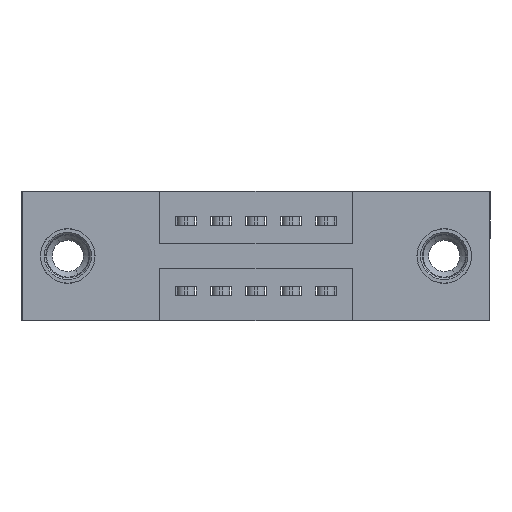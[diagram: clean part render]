
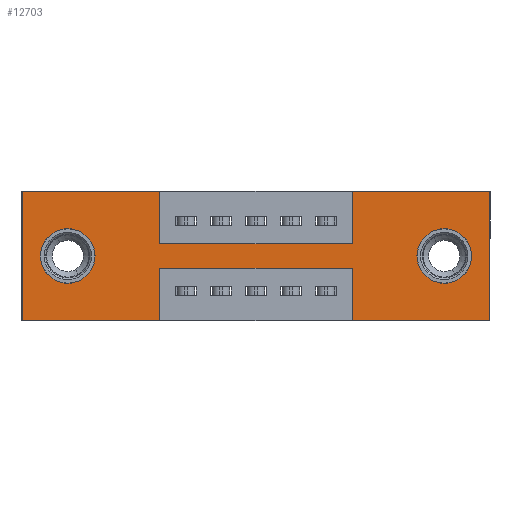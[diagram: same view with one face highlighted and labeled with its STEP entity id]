
A CAD part, front view. The second image highlights one B-rep face of the part: STEP entity #12703.
In plain terms, the highlighted planar face has unit normal (0, -1, 0).
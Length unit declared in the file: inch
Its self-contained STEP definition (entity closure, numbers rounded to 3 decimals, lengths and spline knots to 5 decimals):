
#66 = ORIENTED_EDGE ( 'NONE', *, *, #3494, .F. ) ;
#139 = LINE ( 'NONE', #12505, #10980 ) ;
#207 = DIRECTION ( 'NONE',  ( 0., 1., 0. ) ) ;
#402 = CARTESIAN_POINT ( 'NONE',  ( 0.3925, 0., -0.15 ) ) ;
#464 = ORIENTED_EDGE ( 'NONE', *, *, #2959, .T. ) ;
#584 = CARTESIAN_POINT ( 'NONE',  ( 0., 0., 0. ) ) ;
#816 = CARTESIAN_POINT ( 'NONE',  ( 1.335, 0., -0.37 ) ) ;
#910 = VECTOR ( 'NONE', #1062, 39.37008 ) ;
#927 = LINE ( 'NONE', #5054, #3388 ) ;
#940 = VERTEX_POINT ( 'NONE', #6028 ) ;
#985 = DIRECTION ( 'NONE',  ( 0., 0., -1. ) ) ;
#1062 = DIRECTION ( 'NONE',  ( -1., 0., 0. ) ) ;
#1166 = DIRECTION ( 'NONE',  ( 1., 0., 0. ) ) ;
#1214 = CIRCLE ( 'NONE', #7462, 0.078 ) ;
#1317 = EDGE_CURVE ( 'NONE', #9127, #8757, #927, .T. ) ;
#1395 = VECTOR ( 'NONE', #6409, 39.37008 ) ;
#1417 = VERTEX_POINT ( 'NONE', #12292 ) ;
#1451 = EDGE_CURVE ( 'NONE', #7042, #5371, #3368, .T. ) ;
#1458 = FACE_BOUND ( 'NONE', #3312, .T. ) ;
#1490 = CARTESIAN_POINT ( 'NONE',  ( 1.335, 0., 0. ) ) ;
#1551 = AXIS2_PLACEMENT_3D ( 'NONE', #11576, #4367, #9561 ) ;
#1756 = DIRECTION ( 'NONE',  ( 0., 0., -1. ) ) ;
#1987 = VERTEX_POINT ( 'NONE', #10282 ) ;
#2015 = ORIENTED_EDGE ( 'NONE', *, *, #8600, .F. ) ;
#2095 = VERTEX_POINT ( 'NONE', #2300 ) ;
#2158 = EDGE_CURVE ( 'NONE', #5371, #1417, #6440, .T. ) ;
#2300 = CARTESIAN_POINT ( 'NONE',  ( 0., 0., -0.37 ) ) ;
#2510 = VECTOR ( 'NONE', #7547, 39.37008 ) ;
#2517 = ORIENTED_EDGE ( 'NONE', *, *, #7782, .F. ) ;
#2550 = ORIENTED_EDGE ( 'NONE', *, *, #2588, .F. ) ;
#2588 = EDGE_CURVE ( 'NONE', #3691, #11676, #3673, .T. ) ;
#2832 = CARTESIAN_POINT ( 'NONE',  ( 1.205, 0., -0.107 ) ) ;
#2907 = CARTESIAN_POINT ( 'NONE',  ( 1.205, 0., -0.185 ) ) ;
#2959 = EDGE_CURVE ( 'NONE', #940, #1987, #1214, .T. ) ;
#3046 = VECTOR ( 'NONE', #7233, 39.37008 ) ;
#3155 = VECTOR ( 'NONE', #13037, 39.37008 ) ;
#3312 = EDGE_LOOP ( 'NONE', ( #464, #8197 ) ) ;
#3368 = LINE ( 'NONE', #5937, #8579 ) ;
#3388 = VECTOR ( 'NONE', #12450, 39.37008 ) ;
#3494 = EDGE_CURVE ( 'NONE', #8757, #12376, #10545, .T. ) ;
#3605 = LINE ( 'NONE', #10499, #11149 ) ;
#3608 = EDGE_CURVE ( 'NONE', #6012, #10564, #13182, .T. ) ;
#3673 = LINE ( 'NONE', #12745, #1395 ) ;
#3691 = VERTEX_POINT ( 'NONE', #12827 ) ;
#3743 = PLANE ( 'NONE',  #10872 ) ;
#3776 = VERTEX_POINT ( 'NONE', #2832 ) ;
#3881 = EDGE_CURVE ( 'NONE', #11676, #6012, #12676, .T. ) ;
#4076 = CARTESIAN_POINT ( 'NONE',  ( 1.205, 0., -0.185 ) ) ;
#4189 = DIRECTION ( 'NONE',  ( -1., 0., 0. ) ) ;
#4218 = FACE_BOUND ( 'NONE', #6332, .T. ) ;
#4247 = AXIS2_PLACEMENT_3D ( 'NONE', #4076, #12388, #6031 ) ;
#4367 = DIRECTION ( 'NONE',  ( 0., 1., 0. ) ) ;
#4570 = ORIENTED_EDGE ( 'NONE', *, *, #5522, .F. ) ;
#4667 = EDGE_CURVE ( 'NONE', #5597, #3776, #7029, .T. ) ;
#4749 = DIRECTION ( 'NONE',  ( 0., 0., 1. ) ) ;
#4800 = ORIENTED_EDGE ( 'NONE', *, *, #10953, .T. ) ;
#5054 = CARTESIAN_POINT ( 'NONE',  ( 0.3925, 0., -0.22 ) ) ;
#5285 = CARTESIAN_POINT ( 'NONE',  ( 0.9425, 0., -0.15 ) ) ;
#5371 = VERTEX_POINT ( 'NONE', #816 ) ;
#5380 = CIRCLE ( 'NONE', #1551, 0.078 ) ;
#5448 = VECTOR ( 'NONE', #12685, 39.37008 ) ;
#5522 = EDGE_CURVE ( 'NONE', #12376, #2095, #3605, .T. ) ;
#5597 = VERTEX_POINT ( 'NONE', #5652 ) ;
#5652 = CARTESIAN_POINT ( 'NONE',  ( 1.205, 0., -0.263 ) ) ;
#5726 = LINE ( 'NONE', #7414, #12493 ) ;
#5830 = DIRECTION ( 'NONE',  ( 0., -1., 0. ) ) ;
#5933 = EDGE_CURVE ( 'NONE', #1417, #9127, #139, .T. ) ;
#5937 = CARTESIAN_POINT ( 'NONE',  ( 1.335, 0., 0. ) ) ;
#5967 = EDGE_CURVE ( 'NONE', #1987, #940, #5380, .T. ) ;
#6012 = VERTEX_POINT ( 'NONE', #5285 ) ;
#6028 = CARTESIAN_POINT ( 'NONE',  ( 0.13, 0., -0.107 ) ) ;
#6031 = DIRECTION ( 'NONE',  ( 0., 0., -1. ) ) ;
#6054 = ORIENTED_EDGE ( 'NONE', *, *, #1451, .F. ) ;
#6133 = LINE ( 'NONE', #584, #11917 ) ;
#6138 = DIRECTION ( 'NONE',  ( 0., 0., 1. ) ) ;
#6332 = EDGE_LOOP ( 'NONE', ( #4800, #13461 ) ) ;
#6362 = CARTESIAN_POINT ( 'NONE',  ( 0.9425, 0., 0. ) ) ;
#6409 = DIRECTION ( 'NONE',  ( 0., 0., -1. ) ) ;
#6440 = LINE ( 'NONE', #10510, #910 ) ;
#7029 = CIRCLE ( 'NONE', #4247, 0.078 ) ;
#7042 = VERTEX_POINT ( 'NONE', #1490 ) ;
#7233 = DIRECTION ( 'NONE',  ( 1., 0., 0. ) ) ;
#7251 = ORIENTED_EDGE ( 'NONE', *, *, #2158, .F. ) ;
#7397 = CARTESIAN_POINT ( 'NONE',  ( 0.3925, 0., -0.15 ) ) ;
#7414 = CARTESIAN_POINT ( 'NONE',  ( 0., 0., 0. ) ) ;
#7462 = AXIS2_PLACEMENT_3D ( 'NONE', #8669, #207, #7569 ) ;
#7547 = DIRECTION ( 'NONE',  ( 0., 0., -1. ) ) ;
#7569 = DIRECTION ( 'NONE',  ( 0., 0., 1. ) ) ;
#7764 = CARTESIAN_POINT ( 'NONE',  ( 0., 0., -0.37 ) ) ;
#7782 = EDGE_CURVE ( 'NONE', #2095, #10802, #6133, .T. ) ;
#8059 = CARTESIAN_POINT ( 'NONE',  ( 0., 0., 0. ) ) ;
#8138 = FACE_OUTER_BOUND ( 'NONE', #12334, .T. ) ;
#8186 = CARTESIAN_POINT ( 'NONE',  ( 0.9425, 0., -0.22 ) ) ;
#8197 = ORIENTED_EDGE ( 'NONE', *, *, #5967, .T. ) ;
#8579 = VECTOR ( 'NONE', #1756, 39.37008 ) ;
#8580 = LINE ( 'NONE', #8059, #3046 ) ;
#8600 = EDGE_CURVE ( 'NONE', #10802, #3691, #8580, .T. ) ;
#8669 = CARTESIAN_POINT ( 'NONE',  ( 0.13, 0., -0.185 ) ) ;
#8757 = VERTEX_POINT ( 'NONE', #9595 ) ;
#9127 = VERTEX_POINT ( 'NONE', #8186 ) ;
#9350 = AXIS2_PLACEMENT_3D ( 'NONE', #2907, #13464, #985 ) ;
#9561 = DIRECTION ( 'NONE',  ( 0., 0., 1. ) ) ;
#9595 = CARTESIAN_POINT ( 'NONE',  ( 0.3925, 0., -0.22 ) ) ;
#9641 = ORIENTED_EDGE ( 'NONE', *, *, #3881, .F. ) ;
#9868 = CARTESIAN_POINT ( 'NONE',  ( 0.3925, 0., -0.37 ) ) ;
#10282 = CARTESIAN_POINT ( 'NONE',  ( 0.13, 0., -0.263 ) ) ;
#10499 = CARTESIAN_POINT ( 'NONE',  ( 0., 0., -0.37 ) ) ;
#10510 = CARTESIAN_POINT ( 'NONE',  ( 0., 0., -0.37 ) ) ;
#10545 = LINE ( 'NONE', #9868, #2510 ) ;
#10564 = VERTEX_POINT ( 'NONE', #11674 ) ;
#10802 = VERTEX_POINT ( 'NONE', #12254 ) ;
#10872 = AXIS2_PLACEMENT_3D ( 'NONE', #7764, #5830, #13169 ) ;
#10941 = ORIENTED_EDGE ( 'NONE', *, *, #11121, .F. ) ;
#10953 = EDGE_CURVE ( 'NONE', #3776, #5597, #11494, .T. ) ;
#10980 = VECTOR ( 'NONE', #6138, 39.37008 ) ;
#11027 = CARTESIAN_POINT ( 'NONE',  ( 0.3925, 0., -0.37 ) ) ;
#11121 = EDGE_CURVE ( 'NONE', #10564, #7042, #5726, .T. ) ;
#11149 = VECTOR ( 'NONE', #4189, 39.37008 ) ;
#11494 = CIRCLE ( 'NONE', #9350, 0.078 ) ;
#11576 = CARTESIAN_POINT ( 'NONE',  ( 0.13, 0., -0.185 ) ) ;
#11674 = CARTESIAN_POINT ( 'NONE',  ( 0.9425, 0., 0. ) ) ;
#11676 = VERTEX_POINT ( 'NONE', #402 ) ;
#11861 = ORIENTED_EDGE ( 'NONE', *, *, #5933, .F. ) ;
#11917 = VECTOR ( 'NONE', #4749, 39.37008 ) ;
#12254 = CARTESIAN_POINT ( 'NONE',  ( 0., 0., 0. ) ) ;
#12292 = CARTESIAN_POINT ( 'NONE',  ( 0.9425, 0., -0.37 ) ) ;
#12334 = EDGE_LOOP ( 'NONE', ( #66, #13365, #11861, #7251, #6054, #10941, #12666, #9641, #2550, #2015, #2517, #4570 ) ) ;
#12376 = VERTEX_POINT ( 'NONE', #11027 ) ;
#12388 = DIRECTION ( 'NONE',  ( 0., 1., 0. ) ) ;
#12450 = DIRECTION ( 'NONE',  ( -1., 0., 0. ) ) ;
#12493 = VECTOR ( 'NONE', #1166, 39.37008 ) ;
#12505 = CARTESIAN_POINT ( 'NONE',  ( 0.9425, 0., -0.37 ) ) ;
#12666 = ORIENTED_EDGE ( 'NONE', *, *, #3608, .F. ) ;
#12676 = LINE ( 'NONE', #7397, #3155 ) ;
#12685 = DIRECTION ( 'NONE',  ( 0., 0., 1. ) ) ;
#12703 = ADVANCED_FACE ( 'NONE', ( #4218, #1458, #8138 ), #3743, .T. ) ;
#12745 = CARTESIAN_POINT ( 'NONE',  ( 0.3925, 0., 0. ) ) ;
#12827 = CARTESIAN_POINT ( 'NONE',  ( 0.3925, 0., 0. ) ) ;
#13037 = DIRECTION ( 'NONE',  ( 1., 0., 0. ) ) ;
#13169 = DIRECTION ( 'NONE',  ( 0., 0., -1. ) ) ;
#13182 = LINE ( 'NONE', #6362, #5448 ) ;
#13365 = ORIENTED_EDGE ( 'NONE', *, *, #1317, .F. ) ;
#13461 = ORIENTED_EDGE ( 'NONE', *, *, #4667, .T. ) ;
#13464 = DIRECTION ( 'NONE',  ( 0., 1., 0. ) ) ;
